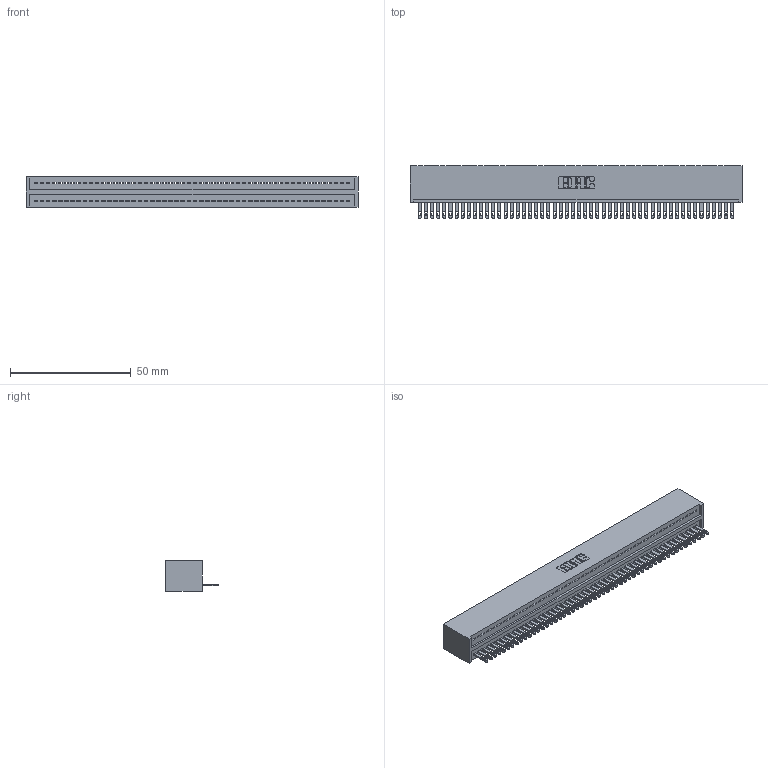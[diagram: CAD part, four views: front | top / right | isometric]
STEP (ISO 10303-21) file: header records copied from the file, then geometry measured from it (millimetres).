
FILE_DESCRIPTION (( 'STEP AP203' ), '1' );
FILE_NAME ('325-052-500-101.STEP', '2020-02-25T00:14:34', ( '' ), ( '' ), 'SwSTEP 2.0', 'SolidWorks 2016', '' );
FILE_SCHEMA (( 'CONFIG_CONTROL_DESIGN' ));
Length unit declared in the file: inch
Products named in the file (3): 325-292-001_325-293-100; 325 Part_Lugless; 325-052-500-101
Assembly tree (53 placements, depth 2):
  325-052-500-101
    325 Part_Lugless
    325-292-001_325-293-100  x52
Bounding box: 137.72 x 21.84 x 12.45 mm (x, y, z)
Volume: 18166 mm3; surface area: 20628.1 mm2
Topology: 53 solids, 53 shells, 2914 faces, 9023 edges, 6014 vertices
Faces by surface type: plane 1938, cylinder 976
Entity records: 30149 total; most frequent: CARTESIAN_POINT 5206, ORIENTED_EDGE 5194, DIRECTION 4365, EDGE_CURVE 2597, VECTOR 2473, LINE 2473, VERTEX_POINT 1730, AXIS2_PLACEMENT_3D 946
